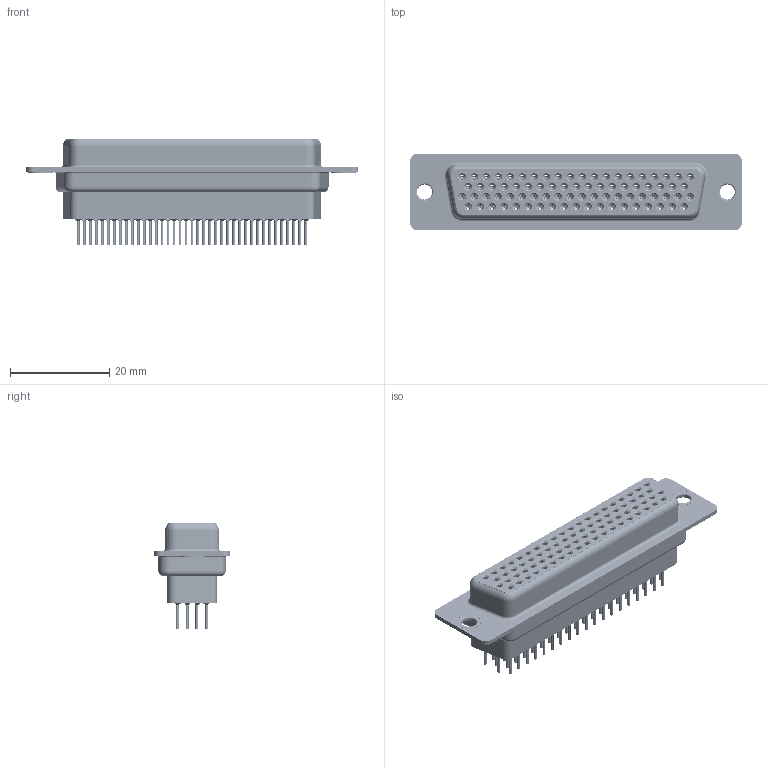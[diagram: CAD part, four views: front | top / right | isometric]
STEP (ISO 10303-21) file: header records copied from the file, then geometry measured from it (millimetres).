
FILE_DESCRIPTION (( 'STEP AP203' ), '1' );
FILE_NAME ('638-078-631-251.STEP', '2020-07-20T04:51:20', ( '' ), ( '' ), 'SwSTEP 2.0', 'SolidWorks 2020', '' );
FILE_SCHEMA (( 'CONFIG_CONTROL_DESIGN' ));
Length unit declared in the file: millimetre
Products named in the file (9): 638 Contact Row 2_31; 638 Shell Rear_78 Contacts; 638 Housing_78 Contacts HP; 638-078-631-251; 638 Shell Front_78 Contacts; 638 Contact Row 3_31; 638 Thru Hole Rivet; 638 Contact Row 78_31; 638 Contact Row 1_31
Assembly tree (83 placements, depth 2):
  638-078-631-251
    638 Housing_78 Contacts HP
    638 Shell Front_78 Contacts
    638 Shell Rear_78 Contacts
    638 Contact Row 1_31  x19
    638 Contact Row 2_31  x20
    638 Contact Row 3_31  x19
    638 Contact Row 78_31  x20
    638 Thru Hole Rivet  x2
Bounding box: 67 x 15.4 x 21.5 mm (x, y, z)
Volume: 7231.4 mm3; surface area: 24867 mm2
Topology: 83 solids, 83 shells, 9847 faces, 25251 edges, 15737 vertices
Faces by surface type: cylinder 2695, plane 2485, torus 1937, bspline 1560, cone 1170
Entity records: 55736 total; most frequent: CARTESIAN_POINT 13050, DIRECTION 8951, ORIENTED_EDGE 7790, EDGE_CURVE 3895, AXIS2_PLACEMENT_3D 3796, VERTEX_POINT 2467, CIRCLE 2103, EDGE_LOOP 2100
